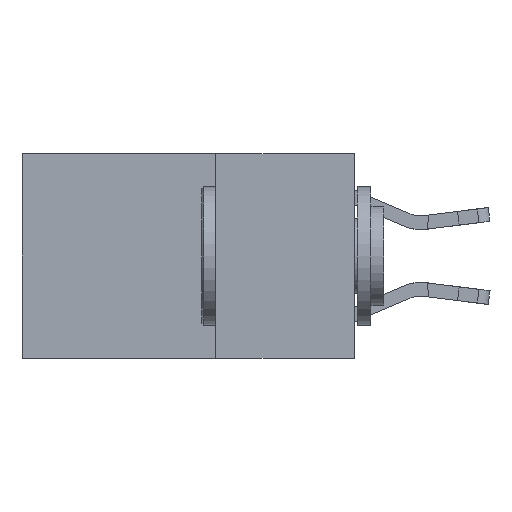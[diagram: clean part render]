
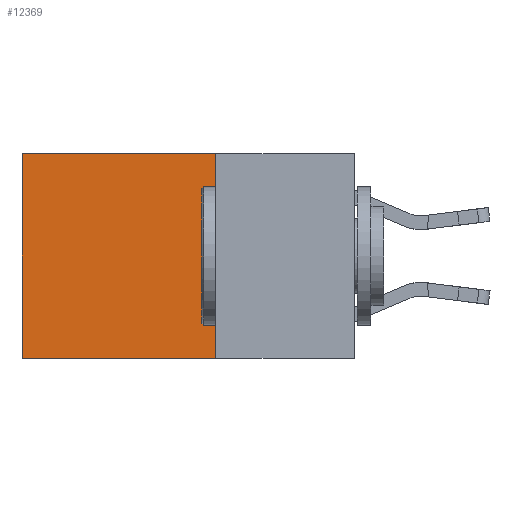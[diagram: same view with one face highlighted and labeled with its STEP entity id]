
A CAD part, left-side view. The second image highlights one B-rep face of the part: STEP entity #12369.
In plain terms, the highlighted planar face has unit normal (-1, 0, 0).
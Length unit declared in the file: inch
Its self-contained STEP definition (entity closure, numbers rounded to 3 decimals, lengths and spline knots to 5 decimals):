
#680 = CARTESIAN_POINT ( 'NONE',  ( 0.2625, 0.25, -0.37 ) ) ;
#761 = DIRECTION ( 'NONE',  ( 0., 1., 0. ) ) ;
#1505 = DIRECTION ( 'NONE',  ( 0., 0., -1. ) ) ;
#1671 = VERTEX_POINT ( 'NONE', #13536 ) ;
#2133 = VECTOR ( 'NONE', #8421, 39.37008 ) ;
#2513 = LINE ( 'NONE', #13116, #2133 ) ;
#2585 = EDGE_CURVE ( 'NONE', #9811, #14636, #3486, .T. ) ;
#2778 = ORIENTED_EDGE ( 'NONE', *, *, #7927, .T. ) ;
#3409 = VECTOR ( 'NONE', #1505, 39.37008 ) ;
#3486 = LINE ( 'NONE', #680, #12646 ) ;
#4724 = CARTESIAN_POINT ( 'NONE',  ( 0.2625, 0.6, 0. ) ) ;
#6039 = CARTESIAN_POINT ( 'NONE',  ( 0.2625, 0.6, 0. ) ) ;
#6176 = ORIENTED_EDGE ( 'NONE', *, *, #8561, .T. ) ;
#6459 = ORIENTED_EDGE ( 'NONE', *, *, #10766, .F. ) ;
#6658 = LINE ( 'NONE', #13478, #3409 ) ;
#6723 = VECTOR ( 'NONE', #14240, 39.37008 ) ;
#7059 = CARTESIAN_POINT ( 'NONE',  ( 0.2625, 0.25, 0. ) ) ;
#7927 = EDGE_CURVE ( 'NONE', #1671, #15353, #2513, .T. ) ;
#8226 = DIRECTION ( 'NONE',  ( 0., 0., -1. ) ) ;
#8421 = DIRECTION ( 'NONE',  ( 0., 1., 0. ) ) ;
#8561 = EDGE_CURVE ( 'NONE', #15353, #14636, #13356, .T. ) ;
#9396 = CARTESIAN_POINT ( 'NONE',  ( 0.2625, 0.6, -0.37 ) ) ;
#9811 = VERTEX_POINT ( 'NONE', #13962 ) ;
#10205 = FACE_OUTER_BOUND ( 'NONE', #11145, .T. ) ;
#10766 = EDGE_CURVE ( 'NONE', #1671, #9811, #6658, .T. ) ;
#11145 = EDGE_LOOP ( 'NONE', ( #6176, #14493, #6459, #2778 ) ) ;
#12369 = ADVANCED_FACE ( 'NONE', ( #10205 ), #14092, .F. ) ;
#12646 = VECTOR ( 'NONE', #761, 39.37008 ) ;
#13116 = CARTESIAN_POINT ( 'NONE',  ( 0.2625, 0.25, 0. ) ) ;
#13356 = LINE ( 'NONE', #6039, #6723 ) ;
#13478 = CARTESIAN_POINT ( 'NONE',  ( 0.2625, 0.25, 0. ) ) ;
#13536 = CARTESIAN_POINT ( 'NONE',  ( 0.2625, 0.25, 0. ) ) ;
#13649 = AXIS2_PLACEMENT_3D ( 'NONE', #7059, #15229, #8226 ) ;
#13962 = CARTESIAN_POINT ( 'NONE',  ( 0.2625, 0.25, -0.37 ) ) ;
#14092 = PLANE ( 'NONE',  #13649 ) ;
#14240 = DIRECTION ( 'NONE',  ( 0., 0., -1. ) ) ;
#14493 = ORIENTED_EDGE ( 'NONE', *, *, #2585, .F. ) ;
#14636 = VERTEX_POINT ( 'NONE', #9396 ) ;
#15229 = DIRECTION ( 'NONE',  ( 1., 0., 0. ) ) ;
#15353 = VERTEX_POINT ( 'NONE', #4724 ) ;
